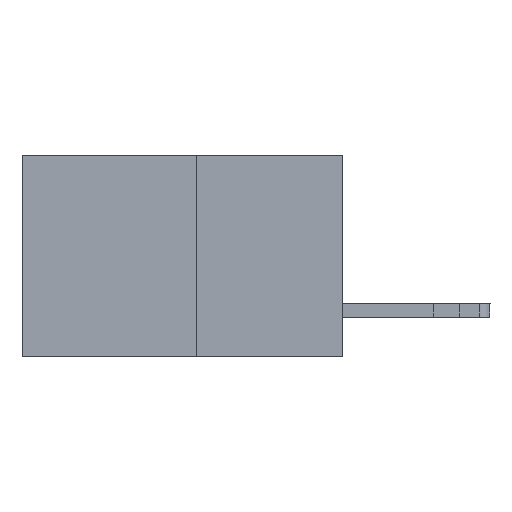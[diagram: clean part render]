
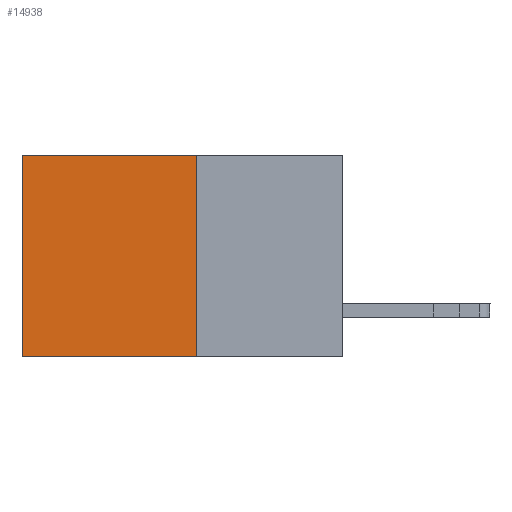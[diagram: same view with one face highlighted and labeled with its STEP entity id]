
A CAD part, left-side view. The second image highlights one B-rep face of the part: STEP entity #14938.
In plain terms, the highlighted planar face has unit normal (-1, 0, 0).
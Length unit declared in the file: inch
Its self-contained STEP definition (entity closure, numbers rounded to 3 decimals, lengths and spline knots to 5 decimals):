
#378 = EDGE_LOOP ( 'NONE', ( #6005, #2607, #8216, #13592 ) ) ;
#394 = CARTESIAN_POINT ( 'NONE',  ( 0.277, 0.59, 0. ) ) ;
#721 = DIRECTION ( 'NONE',  ( 0., 1., 0. ) ) ;
#790 = VERTEX_POINT ( 'NONE', #9659 ) ;
#2303 = CARTESIAN_POINT ( 'NONE',  ( 0.277, 0.59, -0.37 ) ) ;
#2590 = EDGE_CURVE ( 'NONE', #16610, #15184, #12293, .T. ) ;
#2607 = ORIENTED_EDGE ( 'NONE', *, *, #10688, .F. ) ;
#2693 = VECTOR ( 'NONE', #10377, 39.37008 ) ;
#2816 = VECTOR ( 'NONE', #721, 39.37008 ) ;
#2980 = FACE_OUTER_BOUND ( 'NONE', #378, .T. ) ;
#4617 = PLANE ( 'NONE',  #10079 ) ;
#4917 = CARTESIAN_POINT ( 'NONE',  ( 0.277, 0.27, 0. ) ) ;
#5117 = CARTESIAN_POINT ( 'NONE',  ( 0.277, 0.27, -0.37 ) ) ;
#5133 = VECTOR ( 'NONE', #16131, 39.37008 ) ;
#6005 = ORIENTED_EDGE ( 'NONE', *, *, #2590, .T. ) ;
#6021 = DIRECTION ( 'NONE',  ( 0., 0., -1. ) ) ;
#6493 = LINE ( 'NONE', #5117, #17068 ) ;
#8216 = ORIENTED_EDGE ( 'NONE', *, *, #16772, .F. ) ;
#8628 = CARTESIAN_POINT ( 'NONE',  ( 0.277, 0.27, -0.37 ) ) ;
#9049 = CARTESIAN_POINT ( 'NONE',  ( 0.277, 0.27, -0.37 ) ) ;
#9659 = CARTESIAN_POINT ( 'NONE',  ( 0.277, 0.27, -0.37 ) ) ;
#10079 = AXIS2_PLACEMENT_3D ( 'NONE', #8628, #14048, #6021 ) ;
#10377 = DIRECTION ( 'NONE',  ( 0., 0., -1. ) ) ;
#10688 = EDGE_CURVE ( 'NONE', #790, #15184, #6493, .T. ) ;
#11324 = VERTEX_POINT ( 'NONE', #4917 ) ;
#12293 = LINE ( 'NONE', #16147, #5133 ) ;
#12967 = CARTESIAN_POINT ( 'NONE',  ( 0.277, 0.27, 0. ) ) ;
#13562 = LINE ( 'NONE', #9049, #2693 ) ;
#13592 = ORIENTED_EDGE ( 'NONE', *, *, #13839, .T. ) ;
#13839 = EDGE_CURVE ( 'NONE', #11324, #16610, #16729, .T. ) ;
#14048 = DIRECTION ( 'NONE',  ( 1., 0., 0. ) ) ;
#14511 = DIRECTION ( 'NONE',  ( 0., 1., 0. ) ) ;
#14938 = ADVANCED_FACE ( 'NONE', ( #2980 ), #4617, .F. ) ;
#15184 = VERTEX_POINT ( 'NONE', #2303 ) ;
#16131 = DIRECTION ( 'NONE',  ( 0., 0., -1. ) ) ;
#16147 = CARTESIAN_POINT ( 'NONE',  ( 0.277, 0.59, -0.37 ) ) ;
#16610 = VERTEX_POINT ( 'NONE', #394 ) ;
#16729 = LINE ( 'NONE', #12967, #2816 ) ;
#16772 = EDGE_CURVE ( 'NONE', #11324, #790, #13562, .T. ) ;
#17068 = VECTOR ( 'NONE', #14511, 39.37008 ) ;
